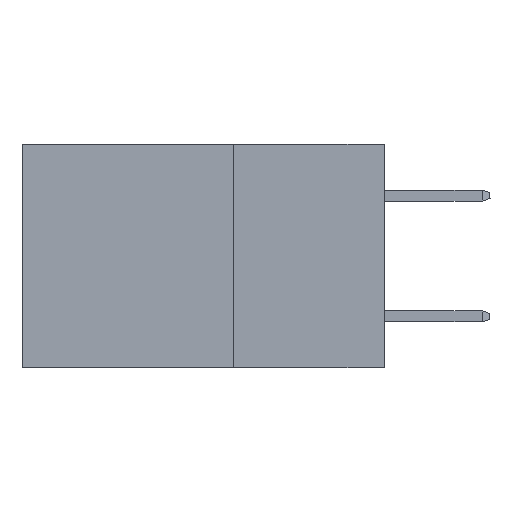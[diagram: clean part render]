
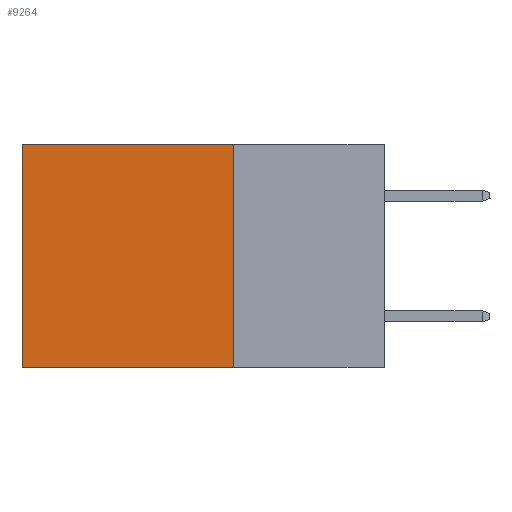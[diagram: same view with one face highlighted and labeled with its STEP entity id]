
A CAD part, left-side view. The second image highlights one B-rep face of the part: STEP entity #9264.
In plain terms, the highlighted planar face has unit normal (-1, 0, 0).
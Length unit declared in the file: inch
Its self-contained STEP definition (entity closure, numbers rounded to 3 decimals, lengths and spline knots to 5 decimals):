
#1457 = EDGE_CURVE ( 'NONE', #10160, #9864, #15397, .T. ) ;
#1755 = ORIENTED_EDGE ( 'NONE', *, *, #6439, .T. ) ;
#2430 = CARTESIAN_POINT ( 'NONE',  ( 0.298, 0.25, 0. ) ) ;
#2629 = CARTESIAN_POINT ( 'NONE',  ( 0.298, 0.25, 0. ) ) ;
#2912 = VECTOR ( 'NONE', #5100, 39.37008 ) ;
#3256 = DIRECTION ( 'NONE',  ( 0., 0., -1. ) ) ;
#4134 = DIRECTION ( 'NONE',  ( 0., 0., -1. ) ) ;
#5100 = DIRECTION ( 'NONE',  ( 0., 1., 0. ) ) ;
#5515 = CARTESIAN_POINT ( 'NONE',  ( 0.298, 0.6, 0. ) ) ;
#5656 = LINE ( 'NONE', #9459, #14913 ) ;
#6145 = DIRECTION ( 'NONE',  ( 0., 1., 0. ) ) ;
#6439 = EDGE_CURVE ( 'NONE', #9114, #7469, #5656, .T. ) ;
#6549 = DIRECTION ( 'NONE',  ( 0., 0., -1. ) ) ;
#7469 = VERTEX_POINT ( 'NONE', #13689 ) ;
#8607 = CARTESIAN_POINT ( 'NONE',  ( 0.298, 0.25, 0. ) ) ;
#9025 = ORIENTED_EDGE ( 'NONE', *, *, #12612, .F. ) ;
#9062 = LINE ( 'NONE', #14866, #2912 ) ;
#9114 = VERTEX_POINT ( 'NONE', #5515 ) ;
#9264 = ADVANCED_FACE ( 'NONE', ( #14792 ), #10471, .F. ) ;
#9459 = CARTESIAN_POINT ( 'NONE',  ( 0.298, 0.6, 0. ) ) ;
#9864 = VERTEX_POINT ( 'NONE', #13366 ) ;
#10160 = VERTEX_POINT ( 'NONE', #2430 ) ;
#10471 = PLANE ( 'NONE',  #15046 ) ;
#10714 = DIRECTION ( 'NONE',  ( 1., 0., 0. ) ) ;
#11160 = EDGE_LOOP ( 'NONE', ( #1755, #9025, #11726, #14074 ) ) ;
#11164 = VECTOR ( 'NONE', #6145, 39.37008 ) ;
#11726 = ORIENTED_EDGE ( 'NONE', *, *, #1457, .F. ) ;
#11863 = VECTOR ( 'NONE', #3256, 39.37008 ) ;
#12612 = EDGE_CURVE ( 'NONE', #9864, #7469, #14265, .T. ) ;
#13366 = CARTESIAN_POINT ( 'NONE',  ( 0.298, 0.25, -0.37 ) ) ;
#13489 = EDGE_CURVE ( 'NONE', #10160, #9114, #9062, .T. ) ;
#13689 = CARTESIAN_POINT ( 'NONE',  ( 0.298, 0.6, -0.37 ) ) ;
#14019 = CARTESIAN_POINT ( 'NONE',  ( 0.298, 0.25, -0.37 ) ) ;
#14074 = ORIENTED_EDGE ( 'NONE', *, *, #13489, .T. ) ;
#14265 = LINE ( 'NONE', #14019, #11164 ) ;
#14792 = FACE_OUTER_BOUND ( 'NONE', #11160, .T. ) ;
#14866 = CARTESIAN_POINT ( 'NONE',  ( 0.298, 0.25, 0. ) ) ;
#14913 = VECTOR ( 'NONE', #4134, 39.37008 ) ;
#15046 = AXIS2_PLACEMENT_3D ( 'NONE', #2629, #10714, #6549 ) ;
#15397 = LINE ( 'NONE', #8607, #11863 ) ;
